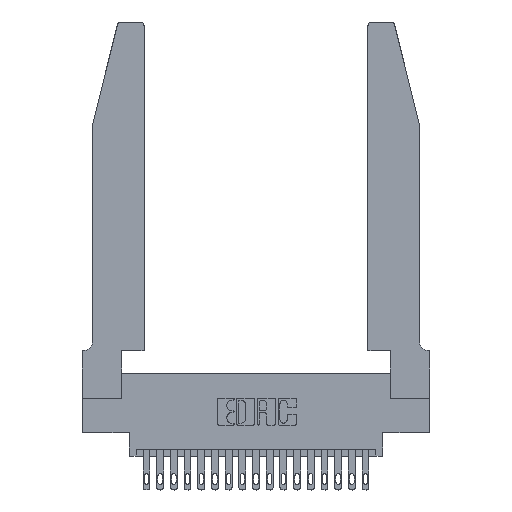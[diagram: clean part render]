
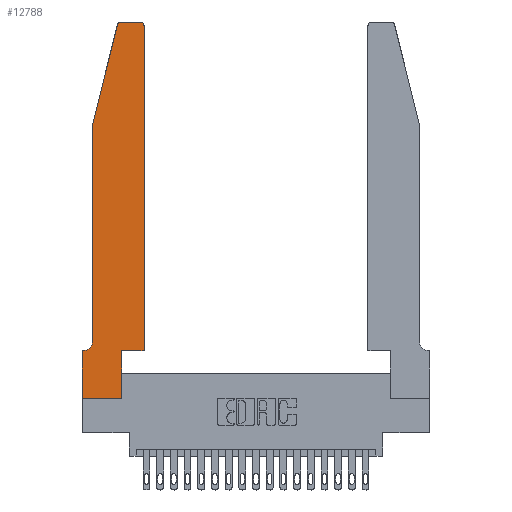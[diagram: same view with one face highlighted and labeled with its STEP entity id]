
A CAD part, top view. The second image highlights one B-rep face of the part: STEP entity #12788.
In plain terms, the highlighted planar face has unit normal (0, 0, 1).
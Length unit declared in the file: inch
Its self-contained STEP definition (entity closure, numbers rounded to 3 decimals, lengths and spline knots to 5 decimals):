
#212 = CARTESIAN_POINT ( 'NONE',  ( 0.2865, 0., 0.37 ) ) ;
#532 = DIRECTION ( 'NONE',  ( -1., 0., 0. ) ) ;
#600 = ORIENTED_EDGE ( 'NONE', *, *, #15846, .T. ) ;
#1352 = VERTEX_POINT ( 'NONE', #10144 ) ;
#1439 = VECTOR ( 'NONE', #15196, 39.37008 ) ;
#1454 = CARTESIAN_POINT ( 'NONE',  ( 0., 0., 0.37 ) ) ;
#1878 = VERTEX_POINT ( 'NONE', #19773 ) ;
#1916 = VERTEX_POINT ( 'NONE', #19625 ) ;
#1947 = CARTESIAN_POINT ( 'NONE',  ( 0.2865, 0.35, 0.37 ) ) ;
#2336 = AXIS2_PLACEMENT_3D ( 'NONE', #7868, #20941, #7945 ) ;
#2674 = CARTESIAN_POINT ( 'NONE',  ( 0., 0., 0.37 ) ) ;
#2787 = CARTESIAN_POINT ( 'NONE',  ( 0.2865, 0.35, 0.37 ) ) ;
#2790 = AXIS2_PLACEMENT_3D ( 'NONE', #9642, #11299, #21336 ) ;
#2884 = DIRECTION ( 'NONE',  ( 1., 0., 0. ) ) ;
#2907 = LINE ( 'NONE', #14132, #6568 ) ;
#2982 = EDGE_CURVE ( 'NONE', #8925, #1916, #7878, .T. ) ;
#3246 = CARTESIAN_POINT ( 'NONE',  ( 0.0755, 2., 0.37 ) ) ;
#3336 = EDGE_CURVE ( 'NONE', #1878, #13229, #8653, .T. ) ;
#3384 = EDGE_CURVE ( 'NONE', #13001, #17070, #6033, .T. ) ;
#3473 = CIRCLE ( 'NONE', #16539, 0.07 ) ;
#3510 = VERTEX_POINT ( 'NONE', #8592 ) ;
#3774 = CARTESIAN_POINT ( 'NONE',  ( 0.284, 2.75, 0.37 ) ) ;
#4501 = CARTESIAN_POINT ( 'NONE',  ( 0.4205, 2.75, 0.37 ) ) ;
#4511 = EDGE_CURVE ( 'NONE', #14478, #8925, #7811, .T. ) ;
#5013 = CARTESIAN_POINT ( 'NONE',  ( 0., 0.35, 0.37 ) ) ;
#5183 = ORIENTED_EDGE ( 'NONE', *, *, #4511, .T. ) ;
#5221 = VECTOR ( 'NONE', #2884, 39.37008 ) ;
#5682 = ORIENTED_EDGE ( 'NONE', *, *, #12381, .T. ) ;
#5739 = LINE ( 'NONE', #21137, #5221 ) ;
#5786 = DIRECTION ( 'NONE',  ( 0., -1., 0. ) ) ;
#6033 = LINE ( 'NONE', #16454, #17197 ) ;
#6557 = CARTESIAN_POINT ( 'NONE',  ( 0.0755, 2., 0.37 ) ) ;
#6568 = VECTOR ( 'NONE', #7579, 39.37008 ) ;
#6910 = ORIENTED_EDGE ( 'NONE', *, *, #3336, .T. ) ;
#7155 = CARTESIAN_POINT ( 'NONE',  ( 0.0055, 0.42, 0.37 ) ) ;
#7579 = DIRECTION ( 'NONE',  ( -1., 0., 0. ) ) ;
#7811 = CIRCLE ( 'NONE', #2336, 0.03 ) ;
#7868 = CARTESIAN_POINT ( 'NONE',  ( 0.284, 2.72, 0.37 ) ) ;
#7878 = LINE ( 'NONE', #6557, #9698 ) ;
#7925 = EDGE_CURVE ( 'NONE', #13472, #3510, #5739, .T. ) ;
#7945 = DIRECTION ( 'NONE',  ( 1., 0., 0. ) ) ;
#8002 = EDGE_CURVE ( 'NONE', #13229, #14478, #11166, .T. ) ;
#8287 = EDGE_CURVE ( 'NONE', #1916, #14440, #12692, .T. ) ;
#8359 = DIRECTION ( 'NONE',  ( 0., 0., 1. ) ) ;
#8592 = CARTESIAN_POINT ( 'NONE',  ( 0.4505, 0.35, 0.37 ) ) ;
#8653 = CIRCLE ( 'NONE', #2790, 0.03 ) ;
#8712 = CARTESIAN_POINT ( 'NONE',  ( 0.2605, 2.75, 0.37 ) ) ;
#8925 = VERTEX_POINT ( 'NONE', #21537 ) ;
#8958 = CARTESIAN_POINT ( 'NONE',  ( 0.4505, 0.35, 0.37 ) ) ;
#8966 = ORIENTED_EDGE ( 'NONE', *, *, #17301, .T. ) ;
#9548 = DIRECTION ( 'NONE',  ( 0., -1., 0. ) ) ;
#9642 = CARTESIAN_POINT ( 'NONE',  ( 0.4205, 2.72, 0.37 ) ) ;
#9698 = VECTOR ( 'NONE', #11430, 39.37008 ) ;
#10144 = CARTESIAN_POINT ( 'NONE',  ( 0.0055, 0.35, 0.37 ) ) ;
#10412 = AXIS2_PLACEMENT_3D ( 'NONE', #5013, #8359, #19847 ) ;
#10498 = DIRECTION ( 'NONE',  ( 0., 0., -1. ) ) ;
#10604 = ORIENTED_EDGE ( 'NONE', *, *, #2982, .T. ) ;
#10804 = DIRECTION ( 'NONE',  ( 0., 1., 0. ) ) ;
#11017 = ORIENTED_EDGE ( 'NONE', *, *, #3384, .T. ) ;
#11166 = LINE ( 'NONE', #8712, #12970 ) ;
#11299 = DIRECTION ( 'NONE',  ( 0., 0., 1. ) ) ;
#11430 = DIRECTION ( 'NONE',  ( -0.239, -0.971, 0. ) ) ;
#11534 = VECTOR ( 'NONE', #10804, 39.37008 ) ;
#12381 = EDGE_CURVE ( 'NONE', #14440, #1352, #3473, .T. ) ;
#12692 = LINE ( 'NONE', #3246, #14284 ) ;
#12788 = ADVANCED_FACE ( 'NONE', ( #17943 ), #18154, .T. ) ;
#12970 = VECTOR ( 'NONE', #15385, 39.37008 ) ;
#13001 = VERTEX_POINT ( 'NONE', #2674 ) ;
#13229 = VERTEX_POINT ( 'NONE', #4501 ) ;
#13472 = VERTEX_POINT ( 'NONE', #2787 ) ;
#14132 = CARTESIAN_POINT ( 'NONE',  ( 0.0755, 0.35, 0.37 ) ) ;
#14284 = VECTOR ( 'NONE', #5786, 39.37008 ) ;
#14440 = VERTEX_POINT ( 'NONE', #18112 ) ;
#14478 = VERTEX_POINT ( 'NONE', #3774 ) ;
#14953 = EDGE_CURVE ( 'NONE', #16087, #13001, #15551, .T. ) ;
#15196 = DIRECTION ( 'NONE',  ( 0., 1., 0. ) ) ;
#15205 = ORIENTED_EDGE ( 'NONE', *, *, #8002, .T. ) ;
#15385 = DIRECTION ( 'NONE',  ( -1., 0., 0. ) ) ;
#15551 = LINE ( 'NONE', #1454, #19455 ) ;
#15846 = EDGE_CURVE ( 'NONE', #17070, #13472, #16552, .T. ) ;
#16087 = VERTEX_POINT ( 'NONE', #19373 ) ;
#16454 = CARTESIAN_POINT ( 'NONE',  ( 0., 0., 0.37 ) ) ;
#16539 = AXIS2_PLACEMENT_3D ( 'NONE', #7155, #10498, #532 ) ;
#16552 = LINE ( 'NONE', #1947, #1439 ) ;
#16987 = LINE ( 'NONE', #8958, #11534 ) ;
#17070 = VERTEX_POINT ( 'NONE', #212 ) ;
#17197 = VECTOR ( 'NONE', #18030, 39.37008 ) ;
#17301 = EDGE_CURVE ( 'NONE', #3510, #1878, #16987, .T. ) ;
#17943 = FACE_OUTER_BOUND ( 'NONE', #19900, .T. ) ;
#17988 = EDGE_CURVE ( 'NONE', #1352, #16087, #2907, .T. ) ;
#18030 = DIRECTION ( 'NONE',  ( 1., 0., 0. ) ) ;
#18112 = CARTESIAN_POINT ( 'NONE',  ( 0.0755, 0.42, 0.37 ) ) ;
#18154 = PLANE ( 'NONE',  #10412 ) ;
#19373 = CARTESIAN_POINT ( 'NONE',  ( 0., 0.35, 0.37 ) ) ;
#19455 = VECTOR ( 'NONE', #9548, 39.37008 ) ;
#19625 = CARTESIAN_POINT ( 'NONE',  ( 0.0755, 2., 0.37 ) ) ;
#19773 = CARTESIAN_POINT ( 'NONE',  ( 0.4505, 2.72, 0.37 ) ) ;
#19832 = ORIENTED_EDGE ( 'NONE', *, *, #14953, .T. ) ;
#19847 = DIRECTION ( 'NONE',  ( 1., 0., 0. ) ) ;
#19900 = EDGE_LOOP ( 'NONE', ( #15205, #5183, #10604, #20423, #5682, #20047, #19832, #11017, #600, #20120, #8966, #6910 ) ) ;
#20047 = ORIENTED_EDGE ( 'NONE', *, *, #17988, .T. ) ;
#20120 = ORIENTED_EDGE ( 'NONE', *, *, #7925, .T. ) ;
#20423 = ORIENTED_EDGE ( 'NONE', *, *, #8287, .T. ) ;
#20941 = DIRECTION ( 'NONE',  ( 0., 0., 1. ) ) ;
#21137 = CARTESIAN_POINT ( 'NONE',  ( 0.4505, 0.35, 0.37 ) ) ;
#21336 = DIRECTION ( 'NONE',  ( 1., 0., 0. ) ) ;
#21537 = CARTESIAN_POINT ( 'NONE',  ( 0.25487, 2.72718, 0.37 ) ) ;
